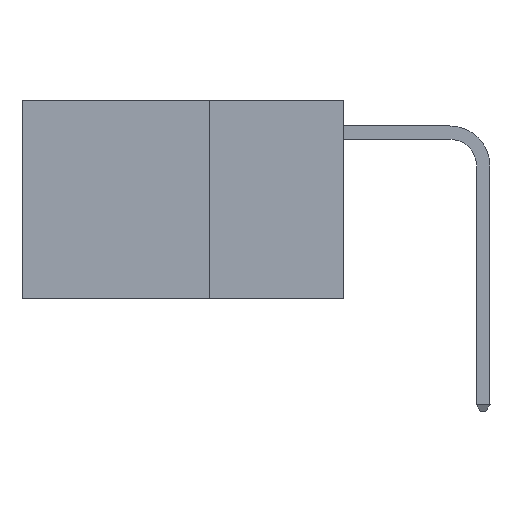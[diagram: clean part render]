
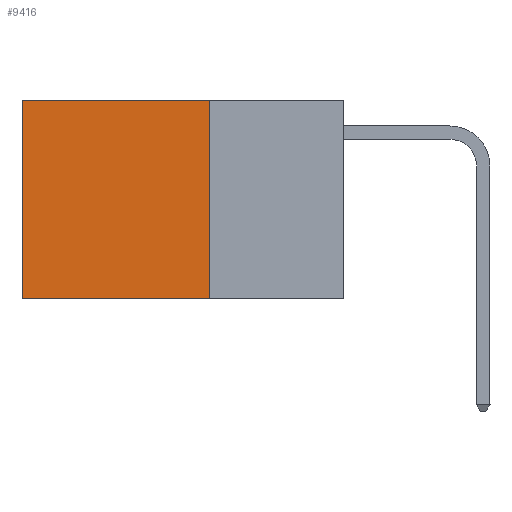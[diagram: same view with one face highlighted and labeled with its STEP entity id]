
A CAD part, left-side view. The second image highlights one B-rep face of the part: STEP entity #9416.
In plain terms, the highlighted planar face has unit normal (-1, 0, 0).
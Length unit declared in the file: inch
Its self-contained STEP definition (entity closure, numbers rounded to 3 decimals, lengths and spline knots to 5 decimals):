
#532 = EDGE_CURVE ( 'NONE', #15163, #4853, #11806, .T. ) ;
#1197 = EDGE_CURVE ( 'NONE', #5244, #9519, #6612, .T. ) ;
#1985 = CARTESIAN_POINT ( 'NONE',  ( 0.2625, 0.25, 0. ) ) ;
#2000 = LINE ( 'NONE', #9042, #12587 ) ;
#2750 = EDGE_LOOP ( 'NONE', ( #9828, #14992, #15582, #6215 ) ) ;
#2978 = DIRECTION ( 'NONE',  ( 0., 0., -1. ) ) ;
#3158 = CARTESIAN_POINT ( 'NONE',  ( 0.2625, 0.6, 0. ) ) ;
#3178 = CARTESIAN_POINT ( 'NONE',  ( 0.2625, 0.25, -0.37 ) ) ;
#3187 = DIRECTION ( 'NONE',  ( 0., 1., 0. ) ) ;
#3415 = DIRECTION ( 'NONE',  ( 0., 1., 0. ) ) ;
#4036 = DIRECTION ( 'NONE',  ( 0., 0., -1. ) ) ;
#4373 = DIRECTION ( 'NONE',  ( 1., 0., 0. ) ) ;
#4564 = FACE_OUTER_BOUND ( 'NONE', #2750, .T. ) ;
#4853 = VERTEX_POINT ( 'NONE', #10165 ) ;
#5244 = VERTEX_POINT ( 'NONE', #17752 ) ;
#5809 = PLANE ( 'NONE',  #10317 ) ;
#5868 = VECTOR ( 'NONE', #2978, 39.37008 ) ;
#5926 = LINE ( 'NONE', #3158, #5868 ) ;
#6151 = CARTESIAN_POINT ( 'NONE',  ( 0.2625, 0.25, 0. ) ) ;
#6215 = ORIENTED_EDGE ( 'NONE', *, *, #532, .T. ) ;
#6612 = LINE ( 'NONE', #3178, #6819 ) ;
#6735 = EDGE_CURVE ( 'NONE', #4853, #9519, #5926, .T. ) ;
#6819 = VECTOR ( 'NONE', #3415, 39.37008 ) ;
#8478 = CARTESIAN_POINT ( 'NONE',  ( 0.2625, 0.25, 0. ) ) ;
#9042 = CARTESIAN_POINT ( 'NONE',  ( 0.2625, 0.25, 0. ) ) ;
#9416 = ADVANCED_FACE ( 'NONE', ( #4564 ), #5809, .F. ) ;
#9519 = VERTEX_POINT ( 'NONE', #11648 ) ;
#9828 = ORIENTED_EDGE ( 'NONE', *, *, #6735, .T. ) ;
#10165 = CARTESIAN_POINT ( 'NONE',  ( 0.2625, 0.6, 0. ) ) ;
#10317 = AXIS2_PLACEMENT_3D ( 'NONE', #6151, #4373, #4036 ) ;
#11586 = VECTOR ( 'NONE', #3187, 39.37008 ) ;
#11648 = CARTESIAN_POINT ( 'NONE',  ( 0.2625, 0.6, -0.37 ) ) ;
#11806 = LINE ( 'NONE', #8478, #11586 ) ;
#12587 = VECTOR ( 'NONE', #15930, 39.37008 ) ;
#14992 = ORIENTED_EDGE ( 'NONE', *, *, #1197, .F. ) ;
#15163 = VERTEX_POINT ( 'NONE', #1985 ) ;
#15582 = ORIENTED_EDGE ( 'NONE', *, *, #17371, .F. ) ;
#15930 = DIRECTION ( 'NONE',  ( 0., 0., -1. ) ) ;
#17371 = EDGE_CURVE ( 'NONE', #15163, #5244, #2000, .T. ) ;
#17752 = CARTESIAN_POINT ( 'NONE',  ( 0.2625, 0.25, -0.37 ) ) ;
